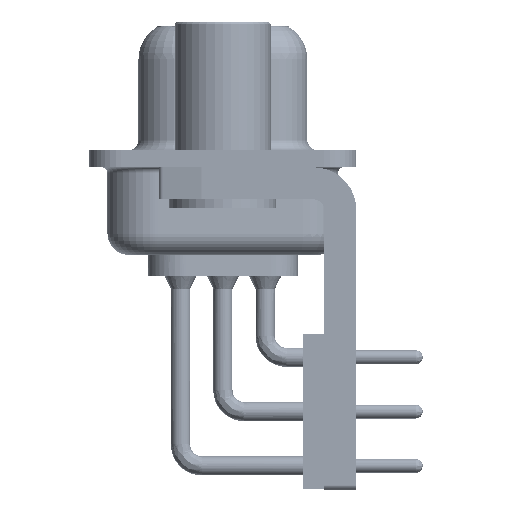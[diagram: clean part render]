
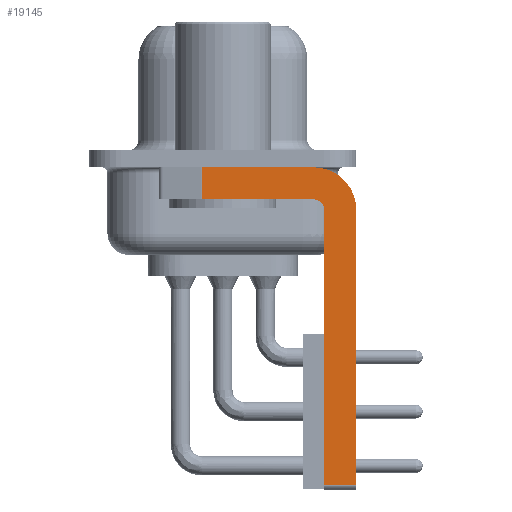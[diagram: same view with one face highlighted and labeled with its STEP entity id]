
A CAD part, left-side view. The second image highlights one B-rep face of the part: STEP entity #19145.
In plain terms, the highlighted planar face has unit normal (-1, 0, 0).
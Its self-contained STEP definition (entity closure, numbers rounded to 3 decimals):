
#107 = CARTESIAN_POINT ( 'NONE',  ( -2.9, -6.25, -15.25 ) ) ;
#449 = CARTESIAN_POINT ( 'NONE',  ( -2.9, 0.978, -1.9 ) ) ;
#1265 = DIRECTION ( 'NONE',  ( 1., 0., 0. ) ) ;
#3172 = DIRECTION ( 'NONE',  ( 0., 0., -1. ) ) ;
#3436 = EDGE_CURVE ( 'NONE', #15245, #43929, #18338, .T. ) ;
#3446 = DIRECTION ( 'NONE',  ( 0., -1., 0. ) ) ;
#5736 = VECTOR ( 'NONE', #36419, 1000. ) ;
#5969 = VERTEX_POINT ( 'NONE', #44713 ) ;
#6524 = CARTESIAN_POINT ( 'NONE',  ( -2.9, -4.25, -2.4 ) ) ;
#7479 = ORIENTED_EDGE ( 'NONE', *, *, #16381, .F. ) ;
#8036 = AXIS2_PLACEMENT_3D ( 'NONE', #22047, #1265, #25554 ) ;
#8325 = VERTEX_POINT ( 'NONE', #12501 ) ;
#8385 = EDGE_CURVE ( 'NONE', #11648, #43929, #23949, .T. ) ;
#8601 = ORIENTED_EDGE ( 'NONE', *, *, #41262, .F. ) ;
#9027 = ORIENTED_EDGE ( 'NONE', *, *, #35313, .F. ) ;
#9162 = CARTESIAN_POINT ( 'NONE',  ( -2.9, -6.25, -2.4 ) ) ;
#9524 = DIRECTION ( 'NONE',  ( 0., 0., -1. ) ) ;
#11423 = VECTOR ( 'NONE', #27112, 1000. ) ;
#11648 = VERTEX_POINT ( 'NONE', #20562 ) ;
#11657 = CARTESIAN_POINT ( 'NONE',  ( -2.9, 0.978, -1.9 ) ) ;
#12479 = AXIS2_PLACEMENT_3D ( 'NONE', #13496, #37733, #16967 ) ;
#12501 = CARTESIAN_POINT ( 'NONE',  ( -2.9, -4.25, -0.4 ) ) ;
#12508 = LINE ( 'NONE', #43909, #11423 ) ;
#12805 = LINE ( 'NONE', #24256, #19869 ) ;
#12963 = CIRCLE ( 'NONE', #8036, 2. ) ;
#13102 = VERTEX_POINT ( 'NONE', #11657 ) ;
#13496 = CARTESIAN_POINT ( 'NONE',  ( -2.9, -4.25, -2.4 ) ) ;
#13618 = CARTESIAN_POINT ( 'NONE',  ( -2.9, 0.978, -0.4 ) ) ;
#15178 = AXIS2_PLACEMENT_3D ( 'NONE', #6524, #23976, #3172 ) ;
#15245 = VERTEX_POINT ( 'NONE', #27277 ) ;
#16381 = EDGE_CURVE ( 'NONE', #39416, #5969, #19219, .T. ) ;
#16967 = DIRECTION ( 'NONE',  ( 0., 0., 1. ) ) ;
#18338 = LINE ( 'NONE', #38130, #27591 ) ;
#19145 = ADVANCED_FACE ( 'NONE', ( #32074 ), #20467, .F. ) ;
#19219 = CIRCLE ( 'NONE', #12479, 0.5 ) ;
#19751 = EDGE_CURVE ( 'NONE', #5969, #13102, #12508, .T. ) ;
#19869 = VECTOR ( 'NONE', #3446, 1000. ) ;
#20467 = PLANE ( 'NONE',  #15178 ) ;
#20562 = CARTESIAN_POINT ( 'NONE',  ( -2.9, -6.25, -2.4 ) ) ;
#21818 = ORIENTED_EDGE ( 'NONE', *, *, #19751, .F. ) ;
#22047 = CARTESIAN_POINT ( 'NONE',  ( -2.9, -4.25, -2.4 ) ) ;
#22668 = CARTESIAN_POINT ( 'NONE',  ( -2.9, -4.75, -15.5 ) ) ;
#23530 = VECTOR ( 'NONE', #31515, 1000. ) ;
#23949 = LINE ( 'NONE', #9162, #41291 ) ;
#23976 = DIRECTION ( 'NONE',  ( 1., 0., 0. ) ) ;
#24256 = CARTESIAN_POINT ( 'NONE',  ( -2.9, 3., -0.4 ) ) ;
#25554 = DIRECTION ( 'NONE',  ( 0., 0., -1. ) ) ;
#27080 = EDGE_LOOP ( 'NONE', ( #9027, #32328, #21818, #7479, #43313, #36219, #43188, #8601 ) ) ;
#27112 = DIRECTION ( 'NONE',  ( 0., 1., 0. ) ) ;
#27277 = CARTESIAN_POINT ( 'NONE',  ( -2.9, -4.75, -15.25 ) ) ;
#27591 = VECTOR ( 'NONE', #38192, 1000. ) ;
#29718 = VERTEX_POINT ( 'NONE', #13618 ) ;
#31515 = DIRECTION ( 'NONE',  ( 0., 0., -1. ) ) ;
#32074 = FACE_OUTER_BOUND ( 'NONE', #27080, .T. ) ;
#32328 = ORIENTED_EDGE ( 'NONE', *, *, #38297, .T. ) ;
#33382 = LINE ( 'NONE', #22668, #5736 ) ;
#35313 = EDGE_CURVE ( 'NONE', #29718, #8325, #12805, .T. ) ;
#36219 = ORIENTED_EDGE ( 'NONE', *, *, #3436, .T. ) ;
#36419 = DIRECTION ( 'NONE',  ( 0., 0., 1. ) ) ;
#37733 = DIRECTION ( 'NONE',  ( -1., 0., 0. ) ) ;
#38130 = CARTESIAN_POINT ( 'NONE',  ( -2.9, -4.25, -15.25 ) ) ;
#38192 = DIRECTION ( 'NONE',  ( 0., -1., 0. ) ) ;
#38297 = EDGE_CURVE ( 'NONE', #29718, #13102, #44117, .T. ) ;
#39416 = VERTEX_POINT ( 'NONE', #41579 ) ;
#41262 = EDGE_CURVE ( 'NONE', #8325, #11648, #12963, .T. ) ;
#41291 = VECTOR ( 'NONE', #9524, 1000. ) ;
#41579 = CARTESIAN_POINT ( 'NONE',  ( -2.9, -4.75, -2.4 ) ) ;
#43188 = ORIENTED_EDGE ( 'NONE', *, *, #8385, .F. ) ;
#43313 = ORIENTED_EDGE ( 'NONE', *, *, #44289, .F. ) ;
#43909 = CARTESIAN_POINT ( 'NONE',  ( -2.9, -4.25, -1.9 ) ) ;
#43929 = VERTEX_POINT ( 'NONE', #107 ) ;
#44117 = LINE ( 'NONE', #449, #23530 ) ;
#44289 = EDGE_CURVE ( 'NONE', #15245, #39416, #33382, .T. ) ;
#44713 = CARTESIAN_POINT ( 'NONE',  ( -2.9, -4.25, -1.9 ) ) ;
